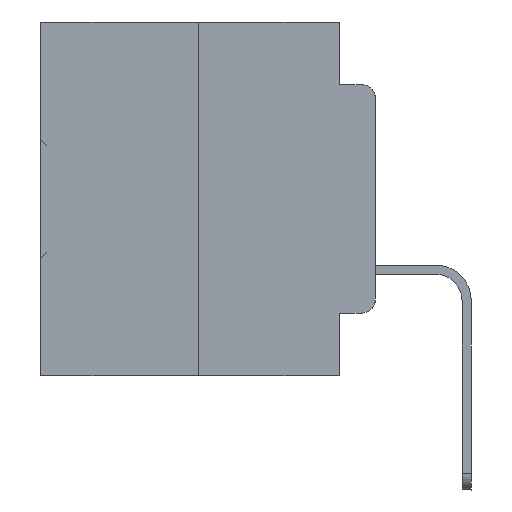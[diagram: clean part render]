
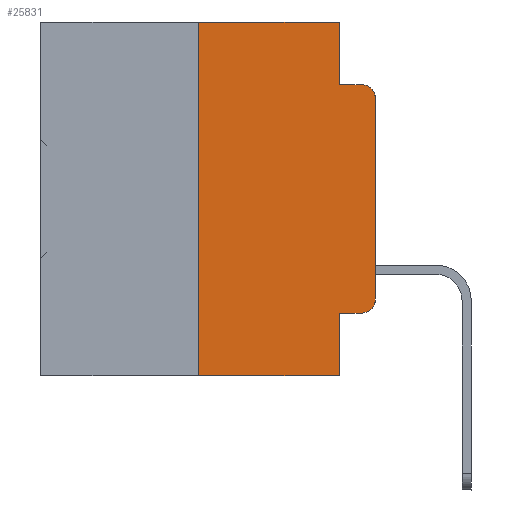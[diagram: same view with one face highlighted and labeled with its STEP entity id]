
A CAD part, left-side view. The second image highlights one B-rep face of the part: STEP entity #25831.
In plain terms, the highlighted planar face has unit normal (-1, 0, 0).
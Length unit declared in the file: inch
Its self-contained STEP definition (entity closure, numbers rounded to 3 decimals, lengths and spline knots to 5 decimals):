
#75 = CARTESIAN_POINT ( 'NONE',  ( 0., 0.051, -0.0885 ) ) ;
#1193 = LINE ( 'NONE', #7938, #27928 ) ;
#1547 = VERTEX_POINT ( 'NONE', #31464 ) ;
#2049 = VERTEX_POINT ( 'NONE', #12620 ) ;
#2078 = VECTOR ( 'NONE', #19307, 39.37008 ) ;
#2098 = ORIENTED_EDGE ( 'NONE', *, *, #13701, .F. ) ;
#2812 = EDGE_CURVE ( 'NONE', #10559, #2049, #25352, .T. ) ;
#2841 = DIRECTION ( 'NONE',  ( 0., -1., 0. ) ) ;
#3997 = DIRECTION ( 'NONE',  ( 0., 0., -1. ) ) ;
#4168 = VECTOR ( 'NONE', #30802, 39.37008 ) ;
#5700 = CARTESIAN_POINT ( 'NONE',  ( 0., 0.473, 0. ) ) ;
#6840 = LINE ( 'NONE', #21263, #2078 ) ;
#6899 = LINE ( 'NONE', #75, #27979 ) ;
#7938 = CARTESIAN_POINT ( 'NONE',  ( 0., 0.051, -0.4115 ) ) ;
#8008 = ORIENTED_EDGE ( 'NONE', *, *, #15963, .T. ) ;
#8271 = VERTEX_POINT ( 'NONE', #29301 ) ;
#8413 = AXIS2_PLACEMENT_3D ( 'NONE', #21462, #15686, #13052 ) ;
#8975 = VECTOR ( 'NONE', #21368, 39.37008 ) ;
#9371 = LINE ( 'NONE', #25384, #4168 ) ;
#10559 = VERTEX_POINT ( 'NONE', #25764 ) ;
#10568 = CARTESIAN_POINT ( 'NONE',  ( 0., 0.473, -0.5 ) ) ;
#10920 = CARTESIAN_POINT ( 'NONE',  ( 0., 0.051, -0.0885 ) ) ;
#11194 = CARTESIAN_POINT ( 'NONE',  ( 0., 0.051, -0.5 ) ) ;
#11410 = CARTESIAN_POINT ( 'NONE',  ( 0., 0.02, -0.0885 ) ) ;
#11664 = AXIS2_PLACEMENT_3D ( 'NONE', #20469, #31819, #3997 ) ;
#11690 = DIRECTION ( 'NONE',  ( 0., 0., 1. ) ) ;
#11774 = CARTESIAN_POINT ( 'NONE',  ( 0., 0.051, 0. ) ) ;
#11962 = LINE ( 'NONE', #15709, #8975 ) ;
#12620 = CARTESIAN_POINT ( 'NONE',  ( 0., 0., -0.3915 ) ) ;
#13052 = DIRECTION ( 'NONE',  ( 0., 0., -1. ) ) ;
#13056 = ORIENTED_EDGE ( 'NONE', *, *, #31374, .F. ) ;
#13451 = DIRECTION ( 'NONE',  ( 0., -1., 0. ) ) ;
#13701 = EDGE_CURVE ( 'NONE', #18272, #16966, #9371, .T. ) ;
#15050 = FACE_OUTER_BOUND ( 'NONE', #28817, .T. ) ;
#15303 = VERTEX_POINT ( 'NONE', #26744 ) ;
#15686 = DIRECTION ( 'NONE',  ( -1., 0., 0. ) ) ;
#15709 = CARTESIAN_POINT ( 'NONE',  ( 0., 0.473, 0. ) ) ;
#15963 = EDGE_CURVE ( 'NONE', #31511, #16966, #26890, .T. ) ;
#16966 = VERTEX_POINT ( 'NONE', #11194 ) ;
#17166 = EDGE_CURVE ( 'NONE', #15303, #26857, #24635, .T. ) ;
#17183 = AXIS2_PLACEMENT_3D ( 'NONE', #5700, #24950, #27723 ) ;
#17708 = CARTESIAN_POINT ( 'NONE',  ( 0., 0., 0. ) ) ;
#18272 = VERTEX_POINT ( 'NONE', #33188 ) ;
#18823 = DIRECTION ( 'NONE',  ( 0., -1., 0. ) ) ;
#19186 = ORIENTED_EDGE ( 'NONE', *, *, #35088, .T. ) ;
#19307 = DIRECTION ( 'NONE',  ( 0., 0., 1. ) ) ;
#19427 = VECTOR ( 'NONE', #30922, 39.37008 ) ;
#20469 = CARTESIAN_POINT ( 'NONE',  ( 0., 0.02, -0.1085 ) ) ;
#21183 = ORIENTED_EDGE ( 'NONE', *, *, #17166, .F. ) ;
#21263 = CARTESIAN_POINT ( 'NONE',  ( 0., 0.25, 0. ) ) ;
#21368 = DIRECTION ( 'NONE',  ( 0., -1., 0. ) ) ;
#21462 = CARTESIAN_POINT ( 'NONE',  ( 0., 0.02, -0.3915 ) ) ;
#22245 = ORIENTED_EDGE ( 'NONE', *, *, #26935, .T. ) ;
#23225 = ORIENTED_EDGE ( 'NONE', *, *, #2812, .T. ) ;
#24635 = LINE ( 'NONE', #11774, #19427 ) ;
#24950 = DIRECTION ( 'NONE',  ( 1., 0., 0. ) ) ;
#25252 = CARTESIAN_POINT ( 'NONE',  ( 0., 0.25, -0.5 ) ) ;
#25352 = CIRCLE ( 'NONE', #8413, 0.02 ) ;
#25384 = CARTESIAN_POINT ( 'NONE',  ( 0., 0.051, 0. ) ) ;
#25764 = CARTESIAN_POINT ( 'NONE',  ( 0., 0.02, -0.4115 ) ) ;
#25831 = ADVANCED_FACE ( 'NONE', ( #15050 ), #33405, .F. ) ;
#26075 = CIRCLE ( 'NONE', #11664, 0.02 ) ;
#26459 = LINE ( 'NONE', #17708, #27323 ) ;
#26744 = CARTESIAN_POINT ( 'NONE',  ( 0., 0.051, 0. ) ) ;
#26857 = VERTEX_POINT ( 'NONE', #10920 ) ;
#26878 = EDGE_CURVE ( 'NONE', #31511, #8271, #6840, .T. ) ;
#26890 = LINE ( 'NONE', #10568, #35568 ) ;
#26935 = EDGE_CURVE ( 'NONE', #18272, #10559, #1193, .T. ) ;
#27323 = VECTOR ( 'NONE', #11690, 39.37008 ) ;
#27723 = DIRECTION ( 'NONE',  ( 0., 0., -1. ) ) ;
#27928 = VECTOR ( 'NONE', #13451, 39.37008 ) ;
#27979 = VECTOR ( 'NONE', #2841, 39.37008 ) ;
#28817 = EDGE_LOOP ( 'NONE', ( #31191, #19186, #13056, #21183, #32130, #29869, #8008, #2098, #22245, #23225 ) ) ;
#29301 = CARTESIAN_POINT ( 'NONE',  ( 0., 0.25, 0. ) ) ;
#29869 = ORIENTED_EDGE ( 'NONE', *, *, #26878, .F. ) ;
#29893 = VERTEX_POINT ( 'NONE', #11410 ) ;
#30802 = DIRECTION ( 'NONE',  ( 0., 0., -1. ) ) ;
#30922 = DIRECTION ( 'NONE',  ( 0., 0., -1. ) ) ;
#30950 = EDGE_CURVE ( 'NONE', #2049, #1547, #26459, .T. ) ;
#31191 = ORIENTED_EDGE ( 'NONE', *, *, #30950, .T. ) ;
#31374 = EDGE_CURVE ( 'NONE', #26857, #29893, #6899, .T. ) ;
#31464 = CARTESIAN_POINT ( 'NONE',  ( 0., 0., -0.1085 ) ) ;
#31511 = VERTEX_POINT ( 'NONE', #25252 ) ;
#31819 = DIRECTION ( 'NONE',  ( -1., 0., 0. ) ) ;
#32130 = ORIENTED_EDGE ( 'NONE', *, *, #32725, .F. ) ;
#32725 = EDGE_CURVE ( 'NONE', #8271, #15303, #11962, .T. ) ;
#33188 = CARTESIAN_POINT ( 'NONE',  ( 0., 0.051, -0.4115 ) ) ;
#33405 = PLANE ( 'NONE',  #17183 ) ;
#35088 = EDGE_CURVE ( 'NONE', #1547, #29893, #26075, .T. ) ;
#35568 = VECTOR ( 'NONE', #18823, 39.37008 ) ;
